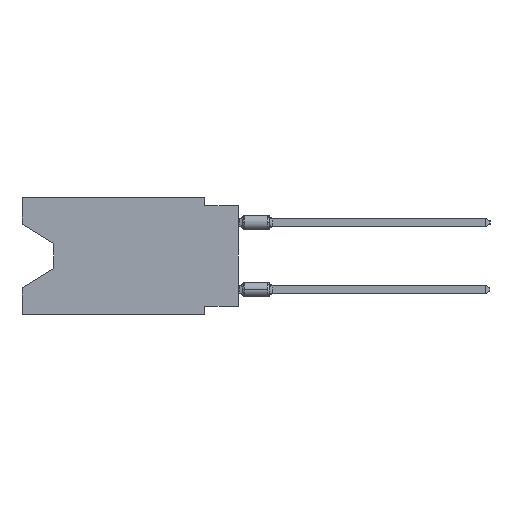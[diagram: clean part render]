
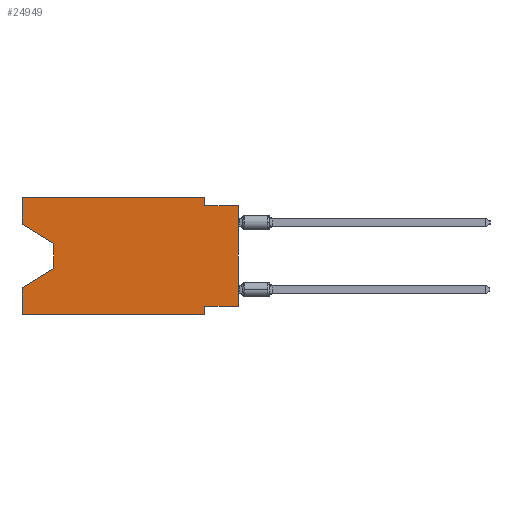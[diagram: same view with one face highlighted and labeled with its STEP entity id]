
A CAD part, left-side view. The second image highlights one B-rep face of the part: STEP entity #24949.
In plain terms, the highlighted planar face has unit normal (-1, 0, 0).
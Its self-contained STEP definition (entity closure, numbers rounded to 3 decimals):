
#645 = CARTESIAN_POINT ( 'NONE',  ( 0., 16.383, -6.852 ) ) ;
#696 = ORIENTED_EDGE ( 'NONE', *, *, #2958, .F. ) ;
#854 = VECTOR ( 'NONE', #36845, 1000. ) ;
#1015 = ORIENTED_EDGE ( 'NONE', *, *, #15307, .F. ) ;
#1147 = FACE_OUTER_BOUND ( 'NONE', #13687, .T. ) ;
#1722 = ORIENTED_EDGE ( 'NONE', *, *, #27823, .T. ) ;
#1760 = ORIENTED_EDGE ( 'NONE', *, *, #31277, .F. ) ;
#1999 = DIRECTION ( 'NONE',  ( 0., 0., 1. ) ) ;
#2907 = LINE ( 'NONE', #34299, #9809 ) ;
#2958 = EDGE_CURVE ( 'NONE', #21293, #18048, #17190, .T. ) ;
#3792 = LINE ( 'NONE', #13427, #35968 ) ;
#4035 = LINE ( 'NONE', #29169, #38386 ) ;
#4124 = CARTESIAN_POINT ( 'NONE',  ( 0., 2.54, -8.89 ) ) ;
#4589 = CARTESIAN_POINT ( 'NONE',  ( 0., 0., -8.255 ) ) ;
#5115 = EDGE_CURVE ( 'NONE', #38777, #18048, #22219, .T. ) ;
#5451 = VERTEX_POINT ( 'NONE', #37431 ) ;
#6753 = DIRECTION ( 'NONE',  ( 0., 0., -1. ) ) ;
#6842 = VECTOR ( 'NONE', #15232, 1000. ) ;
#7190 = DIRECTION ( 'NONE',  ( 0., -1., 0. ) ) ;
#7218 = DIRECTION ( 'NONE',  ( 1., 0., 0. ) ) ;
#7496 = EDGE_CURVE ( 'NONE', #37927, #23769, #30682, .T. ) ;
#8583 = DIRECTION ( 'NONE',  ( 0., -1., 0. ) ) ;
#9069 = CARTESIAN_POINT ( 'NONE',  ( 0., 2.54, 0. ) ) ;
#9222 = VERTEX_POINT ( 'NONE', #34108 ) ;
#9483 = CARTESIAN_POINT ( 'NONE',  ( 0., 2.54, -8.89 ) ) ;
#9809 = VECTOR ( 'NONE', #8583, 1000. ) ;
#10082 = DIRECTION ( 'NONE',  ( 0., 0., -1. ) ) ;
#10362 = CARTESIAN_POINT ( 'NONE',  ( 0., 16.383, 0. ) ) ;
#10378 = CARTESIAN_POINT ( 'NONE',  ( 0., 13.97, -3.505 ) ) ;
#10574 = PLANE ( 'NONE',  #14560 ) ;
#10589 = CARTESIAN_POINT ( 'NONE',  ( 0., 16.383, -2.038 ) ) ;
#10954 = ORIENTED_EDGE ( 'NONE', *, *, #13507, .F. ) ;
#11072 = DIRECTION ( 'NONE',  ( 0., 1., 0. ) ) ;
#11497 = VECTOR ( 'NONE', #12118, 1000. ) ;
#11729 = VECTOR ( 'NONE', #19478, 1000. ) ;
#11735 = VERTEX_POINT ( 'NONE', #9069 ) ;
#12118 = DIRECTION ( 'NONE',  ( 0., 0., 1. ) ) ;
#13161 = EDGE_CURVE ( 'NONE', #29446, #9222, #37838, .T. ) ;
#13427 = CARTESIAN_POINT ( 'NONE',  ( 0., 13.97, -3.505 ) ) ;
#13507 = EDGE_CURVE ( 'NONE', #11735, #40845, #21495, .T. ) ;
#13687 = EDGE_LOOP ( 'NONE', ( #32595, #23877, #34642, #696, #1722, #27700, #1760, #18586, #28006, #10954, #1015, #28259 ) ) ;
#13935 = LINE ( 'NONE', #10589, #22461 ) ;
#14022 = LINE ( 'NONE', #4589, #31685 ) ;
#14560 = AXIS2_PLACEMENT_3D ( 'NONE', #10362, #7218, #38999 ) ;
#15172 = CARTESIAN_POINT ( 'NONE',  ( 0., 13.97, -5.385 ) ) ;
#15232 = DIRECTION ( 'NONE',  ( 0., 0., -1. ) ) ;
#15307 = EDGE_CURVE ( 'NONE', #9222, #11735, #4035, .T. ) ;
#16901 = VECTOR ( 'NONE', #33497, 1000. ) ;
#17190 = LINE ( 'NONE', #26612, #16901 ) ;
#18048 = VERTEX_POINT ( 'NONE', #645 ) ;
#18500 = VERTEX_POINT ( 'NONE', #4124 ) ;
#18586 = ORIENTED_EDGE ( 'NONE', *, *, #7496, .T. ) ;
#19478 = DIRECTION ( 'NONE',  ( 0., 0.855, -0.519 ) ) ;
#20878 = CARTESIAN_POINT ( 'NONE',  ( 0., 2.54, -0.635 ) ) ;
#21293 = VERTEX_POINT ( 'NONE', #22413 ) ;
#21495 = LINE ( 'NONE', #21926, #6842 ) ;
#21770 = CARTESIAN_POINT ( 'NONE',  ( 0., 0., -8.255 ) ) ;
#21926 = CARTESIAN_POINT ( 'NONE',  ( 0., 2.54, 0. ) ) ;
#22099 = EDGE_CURVE ( 'NONE', #5451, #18500, #22465, .T. ) ;
#22219 = LINE ( 'NONE', #15172, #11729 ) ;
#22413 = CARTESIAN_POINT ( 'NONE',  ( 0., 16.383, -8.89 ) ) ;
#22461 = VECTOR ( 'NONE', #29835, 1000. ) ;
#22465 = LINE ( 'NONE', #9483, #26862 ) ;
#22786 = VECTOR ( 'NONE', #1999, 1000. ) ;
#23769 = VERTEX_POINT ( 'NONE', #37521 ) ;
#23877 = ORIENTED_EDGE ( 'NONE', *, *, #37619, .T. ) ;
#23913 = CARTESIAN_POINT ( 'NONE',  ( 0., 16.383, -8.89 ) ) ;
#24949 = ADVANCED_FACE ( 'NONE', ( #1147 ), #10574, .F. ) ;
#26188 = CARTESIAN_POINT ( 'NONE',  ( 0., 16.383, -2.038 ) ) ;
#26612 = CARTESIAN_POINT ( 'NONE',  ( 0., 16.383, 0. ) ) ;
#26862 = VECTOR ( 'NONE', #6753, 1000. ) ;
#27700 = ORIENTED_EDGE ( 'NONE', *, *, #22099, .F. ) ;
#27823 = EDGE_CURVE ( 'NONE', #21293, #18500, #30177, .T. ) ;
#28006 = ORIENTED_EDGE ( 'NONE', *, *, #40559, .F. ) ;
#28259 = ORIENTED_EDGE ( 'NONE', *, *, #13161, .F. ) ;
#28650 = CARTESIAN_POINT ( 'NONE',  ( 0., 16.383, 0. ) ) ;
#29169 = CARTESIAN_POINT ( 'NONE',  ( 0., 16.383, 0. ) ) ;
#29446 = VERTEX_POINT ( 'NONE', #26188 ) ;
#29835 = DIRECTION ( 'NONE',  ( 0., -0.855, -0.519 ) ) ;
#30177 = LINE ( 'NONE', #23913, #854 ) ;
#30682 = LINE ( 'NONE', #30885, #22786 ) ;
#30885 = CARTESIAN_POINT ( 'NONE',  ( 0., 0., 0. ) ) ;
#31277 = EDGE_CURVE ( 'NONE', #37927, #5451, #14022, .T. ) ;
#31685 = VECTOR ( 'NONE', #11072, 1000. ) ;
#32595 = ORIENTED_EDGE ( 'NONE', *, *, #33410, .T. ) ;
#33410 = EDGE_CURVE ( 'NONE', #29446, #33540, #13935, .T. ) ;
#33497 = DIRECTION ( 'NONE',  ( 0., 0., 1. ) ) ;
#33540 = VERTEX_POINT ( 'NONE', #10378 ) ;
#34108 = CARTESIAN_POINT ( 'NONE',  ( 0., 16.383, 0. ) ) ;
#34299 = CARTESIAN_POINT ( 'NONE',  ( 0., 0., -0.635 ) ) ;
#34642 = ORIENTED_EDGE ( 'NONE', *, *, #5115, .T. ) ;
#35194 = CARTESIAN_POINT ( 'NONE',  ( 0., 13.97, -5.385 ) ) ;
#35968 = VECTOR ( 'NONE', #10082, 1000. ) ;
#36845 = DIRECTION ( 'NONE',  ( 0., -1., 0. ) ) ;
#37431 = CARTESIAN_POINT ( 'NONE',  ( 0., 2.54, -8.255 ) ) ;
#37521 = CARTESIAN_POINT ( 'NONE',  ( 0., 0., -0.635 ) ) ;
#37619 = EDGE_CURVE ( 'NONE', #33540, #38777, #3792, .T. ) ;
#37838 = LINE ( 'NONE', #28650, #11497 ) ;
#37927 = VERTEX_POINT ( 'NONE', #21770 ) ;
#38386 = VECTOR ( 'NONE', #7190, 1000. ) ;
#38777 = VERTEX_POINT ( 'NONE', #35194 ) ;
#38999 = DIRECTION ( 'NONE',  ( 0., 0., -1. ) ) ;
#40559 = EDGE_CURVE ( 'NONE', #40845, #23769, #2907, .T. ) ;
#40845 = VERTEX_POINT ( 'NONE', #20878 ) ;
